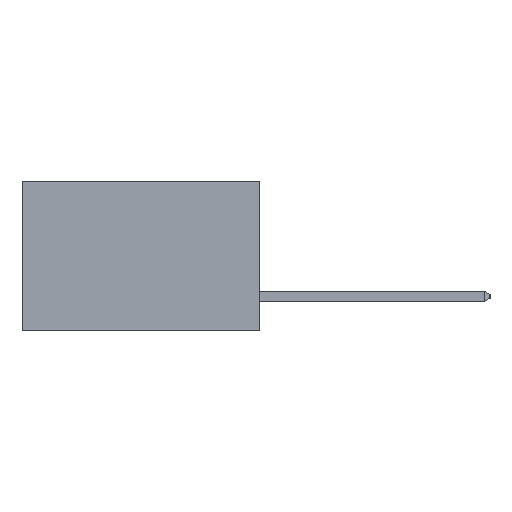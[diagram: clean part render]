
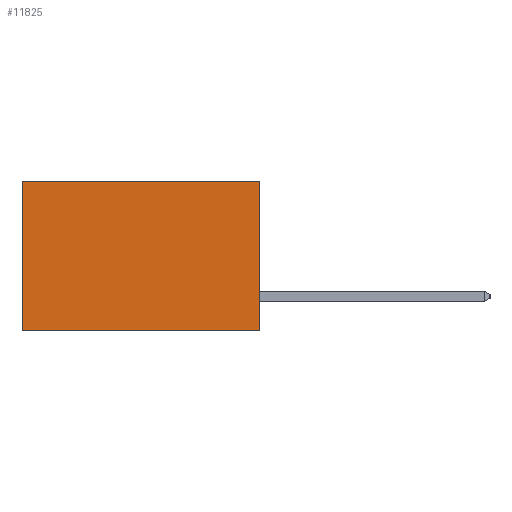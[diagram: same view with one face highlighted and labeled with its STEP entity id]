
A CAD part, left-side view. The second image highlights one B-rep face of the part: STEP entity #11825.
In plain terms, the highlighted planar face has unit normal (-1, 0, 0).
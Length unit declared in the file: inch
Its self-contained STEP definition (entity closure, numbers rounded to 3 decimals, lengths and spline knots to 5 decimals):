
#1582 = VECTOR ( 'NONE', #17402, 39.37008 ) ;
#1845 = EDGE_LOOP ( 'NONE', ( #3556, #16432, #21395, #23224 ) ) ;
#3275 = CARTESIAN_POINT ( 'NONE',  ( 0.277, 0., -0.37 ) ) ;
#3355 = DIRECTION ( 'NONE',  ( 1., 0., 0. ) ) ;
#3556 = ORIENTED_EDGE ( 'NONE', *, *, #21677, .T. ) ;
#8046 = EDGE_CURVE ( 'NONE', #17364, #20134, #13521, .T. ) ;
#9063 = CARTESIAN_POINT ( 'NONE',  ( 0.277, 0., -0.37 ) ) ;
#9158 = VECTOR ( 'NONE', #19111, 39.37008 ) ;
#9601 = VERTEX_POINT ( 'NONE', #23157 ) ;
#10191 = VERTEX_POINT ( 'NONE', #12993 ) ;
#11797 = LINE ( 'NONE', #15628, #1582 ) ;
#11825 = ADVANCED_FACE ( 'NONE', ( #19650 ), #14612, .F. ) ;
#12993 = CARTESIAN_POINT ( 'NONE',  ( 0.277, 0.59, -0.37 ) ) ;
#13521 = LINE ( 'NONE', #17760, #18193 ) ;
#14246 = LINE ( 'NONE', #3275, #14808 ) ;
#14537 = DIRECTION ( 'NONE',  ( 0., 1., 0. ) ) ;
#14612 = PLANE ( 'NONE',  #23331 ) ;
#14808 = VECTOR ( 'NONE', #14537, 39.37008 ) ;
#15168 = EDGE_CURVE ( 'NONE', #17364, #9601, #11797, .T. ) ;
#15628 = CARTESIAN_POINT ( 'NONE',  ( 0.277, 0., 0. ) ) ;
#16387 = DIRECTION ( 'NONE',  ( 0., 0., -1. ) ) ;
#16432 = ORIENTED_EDGE ( 'NONE', *, *, #17382, .F. ) ;
#17364 = VERTEX_POINT ( 'NONE', #19746 ) ;
#17381 = CARTESIAN_POINT ( 'NONE',  ( 0.277, 0.59, -0.37 ) ) ;
#17382 = EDGE_CURVE ( 'NONE', #20134, #10191, #14246, .T. ) ;
#17402 = DIRECTION ( 'NONE',  ( 0., 1., 0. ) ) ;
#17760 = CARTESIAN_POINT ( 'NONE',  ( 0.277, 0., -0.37 ) ) ;
#18193 = VECTOR ( 'NONE', #23059, 39.37008 ) ;
#18751 = LINE ( 'NONE', #17381, #9158 ) ;
#19111 = DIRECTION ( 'NONE',  ( 0., 0., -1. ) ) ;
#19650 = FACE_OUTER_BOUND ( 'NONE', #1845, .T. ) ;
#19746 = CARTESIAN_POINT ( 'NONE',  ( 0.277, 0., 0. ) ) ;
#19774 = CARTESIAN_POINT ( 'NONE',  ( 0.277, 0., -0.37 ) ) ;
#20134 = VERTEX_POINT ( 'NONE', #19774 ) ;
#21395 = ORIENTED_EDGE ( 'NONE', *, *, #8046, .F. ) ;
#21677 = EDGE_CURVE ( 'NONE', #9601, #10191, #18751, .T. ) ;
#23059 = DIRECTION ( 'NONE',  ( 0., 0., -1. ) ) ;
#23157 = CARTESIAN_POINT ( 'NONE',  ( 0.277, 0.59, 0. ) ) ;
#23224 = ORIENTED_EDGE ( 'NONE', *, *, #15168, .T. ) ;
#23331 = AXIS2_PLACEMENT_3D ( 'NONE', #9063, #3355, #16387 ) ;
